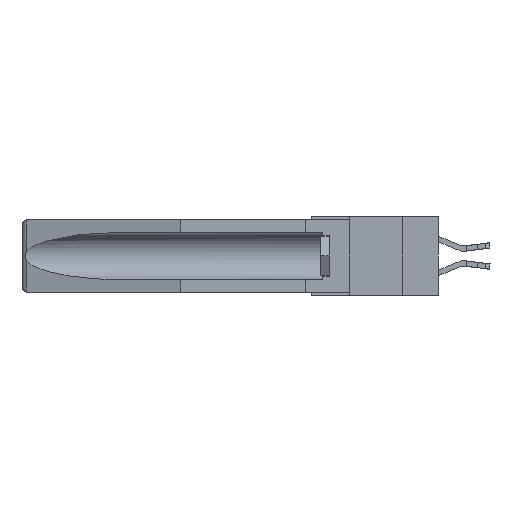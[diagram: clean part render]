
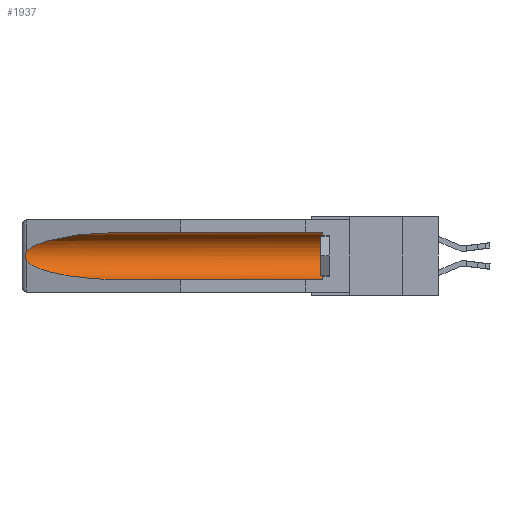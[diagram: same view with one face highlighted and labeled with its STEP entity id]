
A CAD part, left-side view. The second image highlights one B-rep face of the part: STEP entity #1937.
In plain terms, the highlighted cylindrical face has radius 2.857 mm (diameter 5.715 mm), a partial arc.
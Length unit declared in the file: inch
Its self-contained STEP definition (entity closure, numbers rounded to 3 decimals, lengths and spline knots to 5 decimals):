
#364 = AXIS2_PLACEMENT_3D ( 'NONE', #9767, #8404, #12907 ) ;
#787 = EDGE_CURVE ( 'NONE', #11928, #3060, #6054, .T. ) ;
#875 = VECTOR ( 'NONE', #17148, 39.37008 ) ;
#1937 = ADVANCED_FACE ( 'NONE', ( #17064 ), #5089, .F. ) ;
#2000 = VECTOR ( 'NONE', #14774, 39.37008 ) ;
#2384 = CARTESIAN_POINT ( 'NONE',  ( 0.155, 0.126, -0.1715 ) ) ;
#2675 = CARTESIAN_POINT ( 'NONE',  ( 0.26654, 1.53092, -0.15636 ) ) ;
#2682 = EDGE_CURVE ( 'NONE', #14923, #7391, #15244, .T. ) ;
#2902 = CARTESIAN_POINT ( 'NONE',  ( 0.155, 1.07973, -0.284 ) ) ;
#2991 = VERTEX_POINT ( 'NONE', #11943 ) ;
#3060 = VERTEX_POINT ( 'NONE', #13779 ) ;
#3662 = EDGE_CURVE ( 'NONE', #3060, #2991, #12121, .T. ) ;
#4014 = CARTESIAN_POINT ( 'NONE',  ( 0.26597, 1.5296, -0.19026 ) ) ;
#4139 = CARTESIAN_POINT ( 'NONE',  ( 0.2675, 1.53308, -0.16763 ) ) ;
#4230 = CARTESIAN_POINT ( 'NONE',  ( 0.26537, 1.52718, -0.19328 ) ) ;
#4344 = ORIENTED_EDGE ( 'NONE', *, *, #787, .T. ) ;
#4376 = CARTESIAN_POINT ( 'NONE',  ( 0.155, 0.126, -0.059 ) ) ;
#4827 = EDGE_LOOP ( 'NONE', ( #14208, #7016, #11306, #12929, #13487, #4344 ) ) ;
#5089 = CYLINDRICAL_SURFACE ( 'NONE', #364, 0.1125 ) ;
#5132 = VERTEX_POINT ( 'NONE', #14527 ) ;
#5161 = LINE ( 'NONE', #16258, #875 ) ;
#5309 = CARTESIAN_POINT ( 'NONE',  ( 0.155, 1.07973, -0.059 ) ) ;
#5537 = CARTESIAN_POINT ( 'NONE',  ( 0.25451, 1.48313, -0.24835 ) ) ;
#5790 = CARTESIAN_POINT ( 'NONE',  ( 0.155, 1.07973, -0.284 ) ) ;
#6054 = LINE ( 'NONE', #7513, #2000 ) ;
#6882 = CARTESIAN_POINT ( 'NONE',  ( 0.21114, 1.30732, -0.059 ) ) ;
#7013 = CARTESIAN_POINT ( 'NONE',  ( 0.26537, 1.52718, -0.19328 ) ) ;
#7016 = ORIENTED_EDGE ( 'NONE', *, *, #8485, .T. ) ;
#7391 = VERTEX_POINT ( 'NONE', #5790 ) ;
#7513 = CARTESIAN_POINT ( 'NONE',  ( 0.155, -0.30754, -0.059 ) ) ;
#8404 = DIRECTION ( 'NONE',  ( 0., 1., 0. ) ) ;
#8485 = EDGE_CURVE ( 'NONE', #2991, #14923, #15815, .T. ) ;
#8503 = CARTESIAN_POINT ( 'NONE',  ( 0.26537, 1.52718, -0.19328 ) ) ;
#9481 = DIRECTION ( 'NONE',  ( 0., 0., 1. ) ) ;
#9767 = CARTESIAN_POINT ( 'NONE',  ( 0.155, -0.30754, -0.1715 ) ) ;
#9803 = CARTESIAN_POINT ( 'NONE',  ( 0.2675, 1.53308, -0.17534 ) ) ;
#9829 = CARTESIAN_POINT ( 'NONE',  ( 0.21114, 1.30732, -0.284 ) ) ;
#10946 = AXIS2_PLACEMENT_3D ( 'NONE', #2384, #13772, #9481 ) ;
#11035 = CIRCLE ( 'NONE', #10946, 0.1125 ) ;
#11306 = ORIENTED_EDGE ( 'NONE', *, *, #2682, .T. ) ;
#11928 = VERTEX_POINT ( 'NONE', #4376 ) ;
#11943 = CARTESIAN_POINT ( 'NONE',  ( 0.26537, 1.52718, -0.14972 ) ) ;
#12121 =( BOUNDED_CURVE ( )  B_SPLINE_CURVE ( 3, ( #5309, #6882, #12679, #12739 ),
 .UNSPECIFIED., .F., .F. ) 
 B_SPLINE_CURVE_WITH_KNOTS ( ( 4, 4 ),
 ( 4.71239, 6.08839 ),
 .UNSPECIFIED. ) 
 CURVE ( )  GEOMETRIC_REPRESENTATION_ITEM ( )  RATIONAL_B_SPLINE_CURVE ( ( 1., 0.848, 0.848, 1. ) ) 
 REPRESENTATION_ITEM ( '' )  );
#12679 = CARTESIAN_POINT ( 'NONE',  ( 0.25451, 1.48313, -0.09465 ) ) ;
#12739 = CARTESIAN_POINT ( 'NONE',  ( 0.26537, 1.52718, -0.14972 ) ) ;
#12907 = DIRECTION ( 'NONE',  ( 0., 0., 1. ) ) ;
#12929 = ORIENTED_EDGE ( 'NONE', *, *, #15256, .F. ) ;
#13487 = ORIENTED_EDGE ( 'NONE', *, *, #17204, .T. ) ;
#13772 = DIRECTION ( 'NONE',  ( 0., -1., 0. ) ) ;
#13779 = CARTESIAN_POINT ( 'NONE',  ( 0.155, 1.07973, -0.059 ) ) ;
#14016 = CARTESIAN_POINT ( 'NONE',  ( 0.2673, 1.53269, -0.17917 ) ) ;
#14208 = ORIENTED_EDGE ( 'NONE', *, *, #3662, .T. ) ;
#14527 = CARTESIAN_POINT ( 'NONE',  ( 0.155, 0.126, -0.284 ) ) ;
#14774 = DIRECTION ( 'NONE',  ( 0., 1., 0. ) ) ;
#14923 = VERTEX_POINT ( 'NONE', #8503 ) ;
#15244 =( BOUNDED_CURVE ( )  B_SPLINE_CURVE ( 3, ( #4230, #5537, #9829, #2902 ),
 .UNSPECIFIED., .F., .F. ) 
 B_SPLINE_CURVE_WITH_KNOTS ( ( 4, 4 ),
 ( 0.1948, 1.5708 ),
 .UNSPECIFIED. ) 
 CURVE ( )  GEOMETRIC_REPRESENTATION_ITEM ( )  RATIONAL_B_SPLINE_CURVE ( ( 1., 0.848, 0.848, 1. ) ) 
 REPRESENTATION_ITEM ( '' )  );
#15256 = EDGE_CURVE ( 'NONE', #5132, #7391, #5161, .T. ) ;
#15478 = CARTESIAN_POINT ( 'NONE',  ( 0.2673, 1.5327, -0.16383 ) ) ;
#15609 = CARTESIAN_POINT ( 'NONE',  ( 0.26537, 1.52718, -0.14972 ) ) ;
#15815 = B_SPLINE_CURVE_WITH_KNOTS ( 'NONE', 3,
 ( #15609, #17056, #2675, #15478, #4139, #9803, #14016, #18332, #4014, #7013 ),
 .UNSPECIFIED., .F., .F.,
 ( 4, 2, 2, 2, 4 ),
 ( 0., 0.00029, 0.00058, 0.00087, 0.00117 ),
 .UNSPECIFIED. ) ;
#16258 = CARTESIAN_POINT ( 'NONE',  ( 0.155, -0.30754, -0.284 ) ) ;
#17056 = CARTESIAN_POINT ( 'NONE',  ( 0.26597, 1.52961, -0.15275 ) ) ;
#17064 = FACE_OUTER_BOUND ( 'NONE', #4827, .T. ) ;
#17148 = DIRECTION ( 'NONE',  ( 0., 1., 0. ) ) ;
#17204 = EDGE_CURVE ( 'NONE', #5132, #11928, #11035, .T. ) ;
#18332 = CARTESIAN_POINT ( 'NONE',  ( 0.26655, 1.53094, -0.18657 ) ) ;
